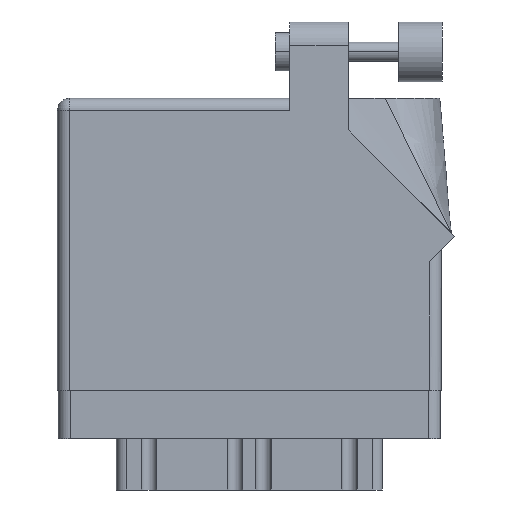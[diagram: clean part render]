
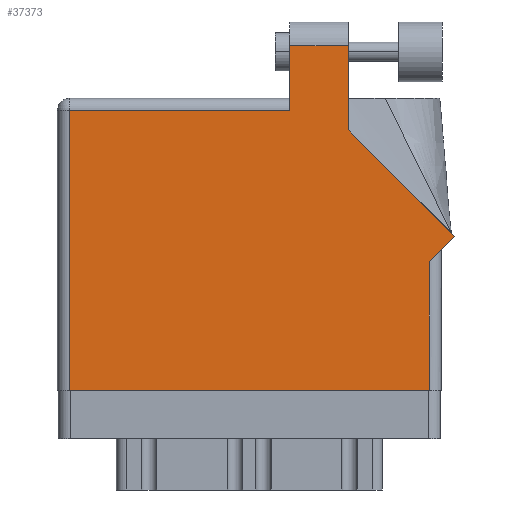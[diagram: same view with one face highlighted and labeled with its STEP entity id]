
A CAD part, front view. The second image highlights one B-rep face of the part: STEP entity #37373.
In plain terms, the highlighted face is planar.
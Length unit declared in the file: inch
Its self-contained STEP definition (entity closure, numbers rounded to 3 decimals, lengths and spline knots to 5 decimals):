
#637 = EDGE_CURVE ( 'NONE', #21267, #9567, #22565, .T. ) ;
#680 = ORIENTED_EDGE ( 'NONE', *, *, #15397, .T. ) ;
#2267 = CARTESIAN_POINT ( 'NONE',  ( 1.948, 0., 0. ) ) ;
#2965 = VECTOR ( 'NONE', #19808, 39.37008 ) ;
#3749 = ORIENTED_EDGE ( 'NONE', *, *, #26774, .T. ) ;
#4111 = CARTESIAN_POINT ( 'NONE',  ( 1.217, 1.805, 0. ) ) ;
#5197 = VECTOR ( 'NONE', #33276, 39.37008 ) ;
#5210 = CARTESIAN_POINT ( 'NONE',  ( 0., 1.468, 0. ) ) ;
#5718 = LINE ( 'NONE', #9021, #30529 ) ;
#6677 = DIRECTION ( 'NONE',  ( 0., 1., 0. ) ) ;
#7068 = DIRECTION ( 'NONE',  ( -1., 0., 0. ) ) ;
#7453 = DIRECTION ( 'NONE',  ( 0., 0., -1. ) ) ;
#8914 = VERTEX_POINT ( 'NONE', #24296 ) ;
#8925 = DIRECTION ( 'NONE',  ( 0., 1., 0. ) ) ;
#9021 = CARTESIAN_POINT ( 'NONE',  ( 1.217, 1.53, 0. ) ) ;
#9245 = ORIENTED_EDGE ( 'NONE', *, *, #21485, .T. ) ;
#9429 = LINE ( 'NONE', #11997, #36739 ) ;
#9567 = VERTEX_POINT ( 'NONE', #13426 ) ;
#9666 = VERTEX_POINT ( 'NONE', #26169 ) ;
#9808 = ORIENTED_EDGE ( 'NONE', *, *, #13962, .T. ) ;
#10289 = EDGE_CURVE ( 'NONE', #23476, #11557, #15090, .T. ) ;
#11557 = VERTEX_POINT ( 'NONE', #4111 ) ;
#11997 = CARTESIAN_POINT ( 'NONE',  ( 1.524, 1.36442, 0. ) ) ;
#12694 = LINE ( 'NONE', #21712, #5197 ) ;
#13172 = PLANE ( 'NONE',  #34777 ) ;
#13426 = CARTESIAN_POINT ( 'NONE',  ( 2.08071, 0.80771, 0. ) ) ;
#13536 = ORIENTED_EDGE ( 'NONE', *, *, #10289, .T. ) ;
#13545 = FACE_OUTER_BOUND ( 'NONE', #29063, .T. ) ;
#13962 = EDGE_CURVE ( 'NONE', #8914, #23476, #9429, .T. ) ;
#14940 = DIRECTION ( 'NONE',  ( 0., -1., 0. ) ) ;
#15090 = LINE ( 'NONE', #33490, #16490 ) ;
#15397 = EDGE_CURVE ( 'NONE', #9666, #19287, #37766, .T. ) ;
#15834 = CARTESIAN_POINT ( 'NONE',  ( 0., 0., 0. ) ) ;
#16490 = VECTOR ( 'NONE', #17511, 39.37008 ) ;
#16807 = DIRECTION ( 'NONE',  ( -1., 0., 0. ) ) ;
#17511 = DIRECTION ( 'NONE',  ( -1., 0., 0. ) ) ;
#19287 = VERTEX_POINT ( 'NONE', #21578 ) ;
#19418 = VECTOR ( 'NONE', #8925, 39.37008 ) ;
#19808 = DIRECTION ( 'NONE',  ( 0.707, 0.707, 0. ) ) ;
#21032 = VECTOR ( 'NONE', #16807, 39.37008 ) ;
#21157 = CARTESIAN_POINT ( 'NONE',  ( 0.062, 0., 0. ) ) ;
#21267 = VERTEX_POINT ( 'NONE', #27793 ) ;
#21485 = EDGE_CURVE ( 'NONE', #32822, #21267, #29726, .T. ) ;
#21578 = CARTESIAN_POINT ( 'NONE',  ( 0.062, 1.468, 0. ) ) ;
#21712 = CARTESIAN_POINT ( 'NONE',  ( 0.062, 0., 0. ) ) ;
#22144 = DIRECTION ( 'NONE',  ( -0.707, 0.707, 0. ) ) ;
#22565 = LINE ( 'NONE', #31376, #2965 ) ;
#23153 = VERTEX_POINT ( 'NONE', #21157 ) ;
#23476 = VERTEX_POINT ( 'NONE', #32272 ) ;
#23535 = VECTOR ( 'NONE', #22144, 39.37008 ) ;
#24078 = DIRECTION ( 'NONE',  ( 1., 0., 0. ) ) ;
#24282 = LINE ( 'NONE', #15834, #30648 ) ;
#24296 = CARTESIAN_POINT ( 'NONE',  ( 1.524, 1.36442, 0. ) ) ;
#24355 = EDGE_CURVE ( 'NONE', #11557, #9666, #5718, .T. ) ;
#24893 = CARTESIAN_POINT ( 'NONE',  ( 2.08071, 0.80771, 0. ) ) ;
#24928 = ORIENTED_EDGE ( 'NONE', *, *, #637, .T. ) ;
#26169 = CARTESIAN_POINT ( 'NONE',  ( 1.217, 1.468, 0. ) ) ;
#26774 = EDGE_CURVE ( 'NONE', #23153, #32822, #24282, .T. ) ;
#27793 = CARTESIAN_POINT ( 'NONE',  ( 1.948, 0.675, 0. ) ) ;
#29063 = EDGE_LOOP ( 'NONE', ( #9808, #13536, #32063, #680, #35387, #3749, #9245, #24928, #32144 ) ) ;
#29726 = LINE ( 'NONE', #32851, #19418 ) ;
#30529 = VECTOR ( 'NONE', #14940, 39.37008 ) ;
#30648 = VECTOR ( 'NONE', #24078, 39.37008 ) ;
#31376 = CARTESIAN_POINT ( 'NONE',  ( 2.01, 0.737, 0. ) ) ;
#32063 = ORIENTED_EDGE ( 'NONE', *, *, #24355, .T. ) ;
#32144 = ORIENTED_EDGE ( 'NONE', *, *, #37837, .T. ) ;
#32272 = CARTESIAN_POINT ( 'NONE',  ( 1.524, 1.805, 0. ) ) ;
#32822 = VERTEX_POINT ( 'NONE', #2267 ) ;
#32851 = CARTESIAN_POINT ( 'NONE',  ( 1.948, 0.737, 0. ) ) ;
#33276 = DIRECTION ( 'NONE',  ( 0., -1., 0. ) ) ;
#33490 = CARTESIAN_POINT ( 'NONE',  ( 1.217, 1.805, 0. ) ) ;
#34334 = CARTESIAN_POINT ( 'NONE',  ( 0., 1.53, 0. ) ) ;
#34710 = EDGE_CURVE ( 'NONE', #19287, #23153, #12694, .T. ) ;
#34777 = AXIS2_PLACEMENT_3D ( 'NONE', #34334, #7453, #7068 ) ;
#35387 = ORIENTED_EDGE ( 'NONE', *, *, #34710, .T. ) ;
#36739 = VECTOR ( 'NONE', #6677, 39.37008 ) ;
#37373 = ADVANCED_FACE ( 'NONE', ( #13545 ), #13172, .F. ) ;
#37417 = LINE ( 'NONE', #24893, #23535 ) ;
#37766 = LINE ( 'NONE', #5210, #21032 ) ;
#37837 = EDGE_CURVE ( 'NONE', #9567, #8914, #37417, .T. ) ;
